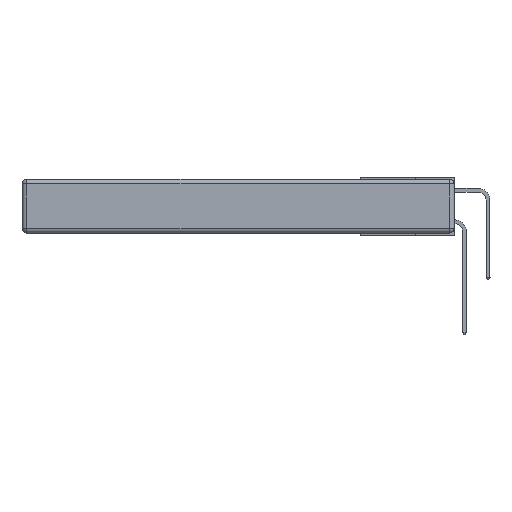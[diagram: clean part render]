
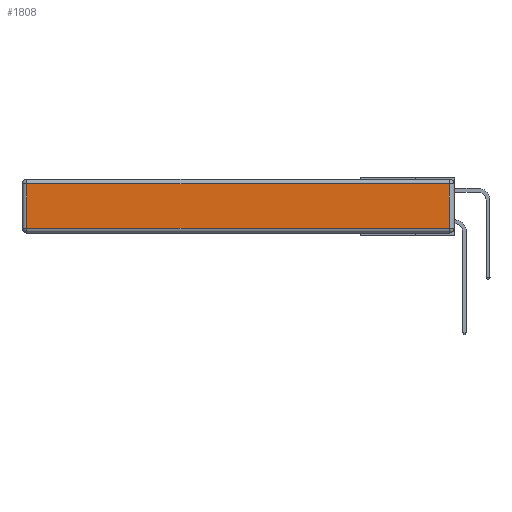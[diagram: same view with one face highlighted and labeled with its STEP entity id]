
A CAD part, left-side view. The second image highlights one B-rep face of the part: STEP entity #1808.
In plain terms, the highlighted planar face has unit normal (-1, 0, 0).
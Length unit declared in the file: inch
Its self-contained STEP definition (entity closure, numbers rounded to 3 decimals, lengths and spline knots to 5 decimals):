
#1555 = DIRECTION ( 'NONE',  ( 0., 0., -1. ) ) ;
#1808 = ADVANCED_FACE ( 'NONE', ( #7014 ), #5704, .T. ) ;
#3283 = CARTESIAN_POINT ( 'NONE',  ( 0., 2.72, -0.343 ) ) ;
#3605 = CARTESIAN_POINT ( 'NONE',  ( 0., 0.03, -0.313 ) ) ;
#4019 = EDGE_CURVE ( 'NONE', #18338, #18770, #17528, .T. ) ;
#4187 = VECTOR ( 'NONE', #1555, 39.37008 ) ;
#5230 = EDGE_CURVE ( 'NONE', #18770, #10454, #7301, .T. ) ;
#5422 = VECTOR ( 'NONE', #18442, 39.37008 ) ;
#5578 = CARTESIAN_POINT ( 'NONE',  ( 0., 0.03, -0.03 ) ) ;
#5704 = PLANE ( 'NONE',  #12029 ) ;
#5710 = CARTESIAN_POINT ( 'NONE',  ( 0., 2.72, -0.313 ) ) ;
#6132 = LINE ( 'NONE', #9696, #11817 ) ;
#7014 = FACE_OUTER_BOUND ( 'NONE', #9250, .T. ) ;
#7168 = CARTESIAN_POINT ( 'NONE',  ( 0., 0., -0.343 ) ) ;
#7301 = LINE ( 'NONE', #12260, #5422 ) ;
#8558 = ORIENTED_EDGE ( 'NONE', *, *, #9122, .T. ) ;
#9122 = EDGE_CURVE ( 'NONE', #10454, #10050, #19309, .T. ) ;
#9250 = EDGE_LOOP ( 'NONE', ( #14154, #8558, #16338, #11722 ) ) ;
#9696 = CARTESIAN_POINT ( 'NONE',  ( 0., 2.75, -0.03 ) ) ;
#10050 = VERTEX_POINT ( 'NONE', #5578 ) ;
#10277 = DIRECTION ( 'NONE',  ( 0., 1., 0. ) ) ;
#10454 = VERTEX_POINT ( 'NONE', #3605 ) ;
#11025 = EDGE_CURVE ( 'NONE', #10050, #18338, #6132, .T. ) ;
#11077 = CARTESIAN_POINT ( 'NONE',  ( 0., 0.03, -0.343 ) ) ;
#11722 = ORIENTED_EDGE ( 'NONE', *, *, #4019, .T. ) ;
#11817 = VECTOR ( 'NONE', #10277, 39.37008 ) ;
#12029 = AXIS2_PLACEMENT_3D ( 'NONE', #7168, #18062, #16548 ) ;
#12260 = CARTESIAN_POINT ( 'NONE',  ( 0., 0., -0.313 ) ) ;
#13956 = DIRECTION ( 'NONE',  ( 0., 0., 1. ) ) ;
#14154 = ORIENTED_EDGE ( 'NONE', *, *, #5230, .T. ) ;
#16338 = ORIENTED_EDGE ( 'NONE', *, *, #11025, .T. ) ;
#16548 = DIRECTION ( 'NONE',  ( 0., 0., 1. ) ) ;
#16702 = VECTOR ( 'NONE', #13956, 39.37008 ) ;
#16837 = CARTESIAN_POINT ( 'NONE',  ( 0., 2.72, -0.03 ) ) ;
#17528 = LINE ( 'NONE', #3283, #4187 ) ;
#18062 = DIRECTION ( 'NONE',  ( -1., 0., 0. ) ) ;
#18338 = VERTEX_POINT ( 'NONE', #16837 ) ;
#18442 = DIRECTION ( 'NONE',  ( 0., -1., 0. ) ) ;
#18770 = VERTEX_POINT ( 'NONE', #5710 ) ;
#19309 = LINE ( 'NONE', #11077, #16702 ) ;
